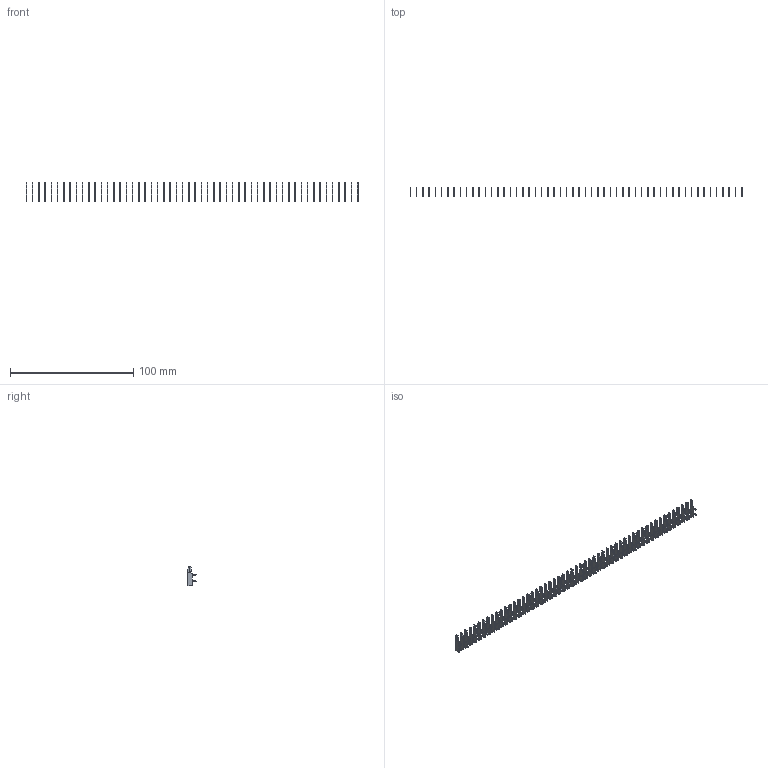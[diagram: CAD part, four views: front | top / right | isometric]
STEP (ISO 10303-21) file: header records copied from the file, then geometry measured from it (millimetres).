
FILE_DESCRIPTION (( 'STEP AP203' ), '1' );
FILE_NAME ('105-054-202-200.STEP', '2020-04-08T00:37:32', ( '' ), ( '' ), 'SwSTEP 2.0', 'SolidWorks 2016', '' );
FILE_SCHEMA (( 'CONFIG_CONTROL_DESIGN' ));
Length unit declared in the file: inch
Products named in the file (2): 105-054-202-200; 100-290-001_100-290-202
Assembly tree (54 placements, depth 2):
  105-054-202-200
    100-290-001_100-290-202  x54
Bounding box: 269.84 x 6.53 x 15.88 mm (x, y, z)
Volume: 1715.7 mm3; surface area: 7630.2 mm2
Topology: 54 solids, 54 shells, 1620 faces, 4536 edges, 3024 vertices
Faces by surface type: plane 1242, cylinder 378
Entity records: 2858 total; most frequent: DIRECTION 268, CARTESIAN_POINT 239, ORIENTED_EDGE 168, LOCAL_TIME 118, COORDINATED_UNIVERSAL_TIME_OFFSET 118, DATE_AND_TIME 118, CALENDAR_DATE 118, AXIS2_PLACEMENT_3D 101
